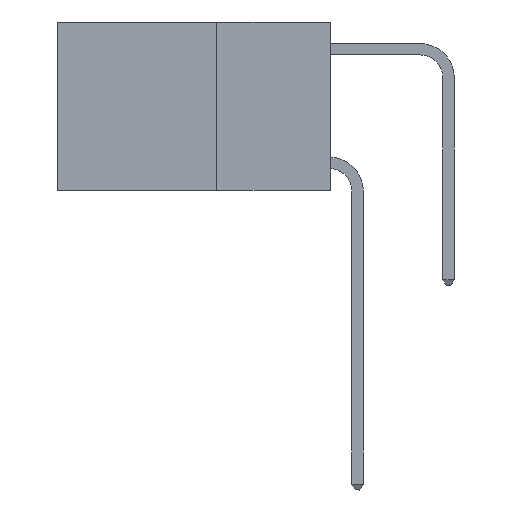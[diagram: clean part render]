
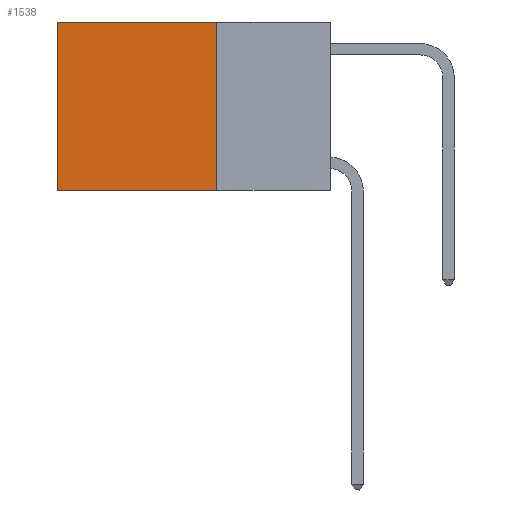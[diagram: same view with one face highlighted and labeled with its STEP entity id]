
A CAD part, left-side view. The second image highlights one B-rep face of the part: STEP entity #1538.
In plain terms, the highlighted planar face has unit normal (-1, 0, 0).
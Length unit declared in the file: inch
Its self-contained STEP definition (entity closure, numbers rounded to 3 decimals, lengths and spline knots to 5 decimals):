
#344 = DIRECTION ( 'NONE',  ( 0., 0., -1. ) ) ;
#729 = ORIENTED_EDGE ( 'NONE', *, *, #2373, .F. ) ;
#1154 = ORIENTED_EDGE ( 'NONE', *, *, #5619, .T. ) ;
#1200 = VECTOR ( 'NONE', #1974, 39.37008 ) ;
#1262 = VECTOR ( 'NONE', #10820, 39.37008 ) ;
#1527 = VERTEX_POINT ( 'NONE', #9079 ) ;
#1538 = ADVANCED_FACE ( 'NONE', ( #8843 ), #9065, .F. ) ;
#1716 = ORIENTED_EDGE ( 'NONE', *, *, #9858, .F. ) ;
#1897 = AXIS2_PLACEMENT_3D ( 'NONE', #9365, #9004, #8976 ) ;
#1974 = DIRECTION ( 'NONE',  ( 0., 1., 0. ) ) ;
#2141 = VERTEX_POINT ( 'NONE', #2982 ) ;
#2373 = EDGE_CURVE ( 'NONE', #10281, #1527, #3616, .T. ) ;
#2982 = CARTESIAN_POINT ( 'NONE',  ( 0.2625, 0.25, 0. ) ) ;
#3038 = VECTOR ( 'NONE', #344, 39.37008 ) ;
#3449 = CARTESIAN_POINT ( 'NONE',  ( 0.2625, 0.25, 0. ) ) ;
#3616 = LINE ( 'NONE', #7487, #1262 ) ;
#4053 = LINE ( 'NONE', #3449, #10383 ) ;
#5499 = LINE ( 'NONE', #10566, #3038 ) ;
#5577 = CARTESIAN_POINT ( 'NONE',  ( 0.2625, 0.6, 0. ) ) ;
#5619 = EDGE_CURVE ( 'NONE', #5621, #1527, #5499, .T. ) ;
#5621 = VERTEX_POINT ( 'NONE', #5577 ) ;
#6905 = EDGE_CURVE ( 'NONE', #2141, #5621, #8514, .T. ) ;
#7014 = CARTESIAN_POINT ( 'NONE',  ( 0.2625, 0.25, 0. ) ) ;
#7487 = CARTESIAN_POINT ( 'NONE',  ( 0.2625, 0.25, -0.37 ) ) ;
#8514 = LINE ( 'NONE', #7014, #1200 ) ;
#8843 = FACE_OUTER_BOUND ( 'NONE', #9336, .T. ) ;
#8976 = DIRECTION ( 'NONE',  ( 0., 0., -1. ) ) ;
#9004 = DIRECTION ( 'NONE',  ( 1., 0., 0. ) ) ;
#9065 = PLANE ( 'NONE',  #1897 ) ;
#9079 = CARTESIAN_POINT ( 'NONE',  ( 0.2625, 0.6, -0.37 ) ) ;
#9336 = EDGE_LOOP ( 'NONE', ( #1154, #729, #1716, #10233 ) ) ;
#9365 = CARTESIAN_POINT ( 'NONE',  ( 0.2625, 0.25, 0. ) ) ;
#9858 = EDGE_CURVE ( 'NONE', #2141, #10281, #4053, .T. ) ;
#10107 = DIRECTION ( 'NONE',  ( 0., 0., -1. ) ) ;
#10233 = ORIENTED_EDGE ( 'NONE', *, *, #6905, .T. ) ;
#10281 = VERTEX_POINT ( 'NONE', #10469 ) ;
#10383 = VECTOR ( 'NONE', #10107, 39.37008 ) ;
#10469 = CARTESIAN_POINT ( 'NONE',  ( 0.2625, 0.25, -0.37 ) ) ;
#10566 = CARTESIAN_POINT ( 'NONE',  ( 0.2625, 0.6, 0. ) ) ;
#10820 = DIRECTION ( 'NONE',  ( 0., 1., 0. ) ) ;
